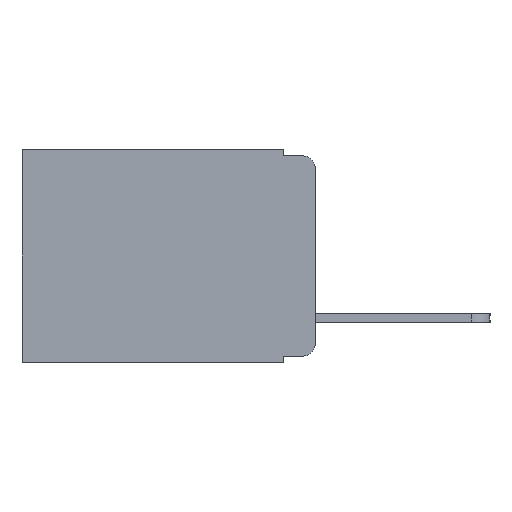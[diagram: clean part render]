
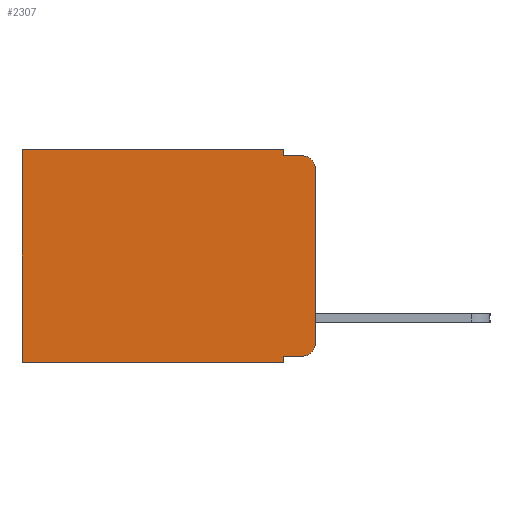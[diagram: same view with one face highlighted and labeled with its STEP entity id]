
A CAD part, left-side view. The second image highlights one B-rep face of the part: STEP entity #2307.
In plain terms, the highlighted planar face has unit normal (-1, 0, 0).
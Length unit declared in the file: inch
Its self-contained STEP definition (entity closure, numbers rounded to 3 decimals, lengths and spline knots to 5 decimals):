
#238 = CARTESIAN_POINT ( 'NONE',  ( 0.298, 0., 0. ) ) ;
#372 = VERTEX_POINT ( 'NONE', #7127 ) ;
#627 = DIRECTION ( 'NONE',  ( 0., 0., -1. ) ) ;
#700 = CARTESIAN_POINT ( 'NONE',  ( 0.298, 0.02, -0.03 ) ) ;
#803 = ORIENTED_EDGE ( 'NONE', *, *, #5936, .T. ) ;
#814 = EDGE_CURVE ( 'NONE', #4172, #1326, #2191, .T. ) ;
#929 = CARTESIAN_POINT ( 'NONE',  ( 0.298, 0.473, -0.343 ) ) ;
#932 = ORIENTED_EDGE ( 'NONE', *, *, #12882, .T. ) ;
#1138 = CARTESIAN_POINT ( 'NONE',  ( 0.298, 0.051, -0.333 ) ) ;
#1326 = VERTEX_POINT ( 'NONE', #11795 ) ;
#1337 = CIRCLE ( 'NONE', #1588, 0.02 ) ;
#1414 = VECTOR ( 'NONE', #9868, 39.37008 ) ;
#1460 = CARTESIAN_POINT ( 'NONE',  ( 0.298, 0.473, 0. ) ) ;
#1588 = AXIS2_PLACEMENT_3D ( 'NONE', #700, #6025, #6030 ) ;
#2191 = LINE ( 'NONE', #16276, #13257 ) ;
#2288 = EDGE_LOOP ( 'NONE', ( #4016, #4283, #4081, #4020, #5687, #7253, #7400, #7434, #803, #932 ) ) ;
#2307 = ADVANCED_FACE ( 'NONE', ( #2395 ), #15409, .F. ) ;
#2395 = FACE_OUTER_BOUND ( 'NONE', #2288, .T. ) ;
#2563 = VECTOR ( 'NONE', #11891, 39.37008 ) ;
#3158 = VECTOR ( 'NONE', #16912, 39.37008 ) ;
#3178 = VERTEX_POINT ( 'NONE', #10220 ) ;
#3566 = CARTESIAN_POINT ( 'NONE',  ( 0.298, 0.051, -0.01 ) ) ;
#3858 = VERTEX_POINT ( 'NONE', #9450 ) ;
#3864 = EDGE_CURVE ( 'NONE', #1326, #13881, #12593, .T. ) ;
#4016 = ORIENTED_EDGE ( 'NONE', *, *, #4179, .F. ) ;
#4020 = ORIENTED_EDGE ( 'NONE', *, *, #7780, .F. ) ;
#4081 = ORIENTED_EDGE ( 'NONE', *, *, #10175, .F. ) ;
#4172 = VERTEX_POINT ( 'NONE', #6106 ) ;
#4179 = EDGE_CURVE ( 'NONE', #15504, #3178, #4556, .T. ) ;
#4283 = ORIENTED_EDGE ( 'NONE', *, *, #5655, .T. ) ;
#4556 = LINE ( 'NONE', #9999, #7911 ) ;
#4930 = AXIS2_PLACEMENT_3D ( 'NONE', #238, #13393, #14440 ) ;
#5003 = DIRECTION ( 'NONE',  ( 0., 1., 0. ) ) ;
#5655 = EDGE_CURVE ( 'NONE', #15504, #3858, #1337, .T. ) ;
#5687 = ORIENTED_EDGE ( 'NONE', *, *, #814, .T. ) ;
#5936 = EDGE_CURVE ( 'NONE', #6296, #372, #6985, .T. ) ;
#6025 = DIRECTION ( 'NONE',  ( -1., 0., 0. ) ) ;
#6030 = DIRECTION ( 'NONE',  ( 0., 0., -1. ) ) ;
#6106 = CARTESIAN_POINT ( 'NONE',  ( 0.298, 0.051, 0. ) ) ;
#6243 = LINE ( 'NONE', #7939, #16553 ) ;
#6296 = VERTEX_POINT ( 'NONE', #1138 ) ;
#6985 = LINE ( 'NONE', #10076, #3158 ) ;
#7100 = EDGE_CURVE ( 'NONE', #6296, #12480, #15959, .T. ) ;
#7127 = CARTESIAN_POINT ( 'NONE',  ( 0.298, 0.02, -0.333 ) ) ;
#7253 = ORIENTED_EDGE ( 'NONE', *, *, #3864, .T. ) ;
#7400 = ORIENTED_EDGE ( 'NONE', *, *, #15795, .F. ) ;
#7434 = ORIENTED_EDGE ( 'NONE', *, *, #7100, .F. ) ;
#7780 = EDGE_CURVE ( 'NONE', #4172, #11171, #6243, .T. ) ;
#7826 = DIRECTION ( 'NONE',  ( 0., 1., 0. ) ) ;
#7899 = CARTESIAN_POINT ( 'NONE',  ( 0.298, 0.051, 0. ) ) ;
#7911 = VECTOR ( 'NONE', #9103, 39.37008 ) ;
#7939 = CARTESIAN_POINT ( 'NONE',  ( 0.298, 0.051, 0. ) ) ;
#8819 = VECTOR ( 'NONE', #14677, 39.37008 ) ;
#9103 = DIRECTION ( 'NONE',  ( 0., 0., -1. ) ) ;
#9143 = DIRECTION ( 'NONE',  ( -1., 0., 0. ) ) ;
#9268 = DIRECTION ( 'NONE',  ( 0., 0., -1. ) ) ;
#9450 = CARTESIAN_POINT ( 'NONE',  ( 0.298, 0.02, -0.01 ) ) ;
#9868 = DIRECTION ( 'NONE',  ( 0., 0., -1. ) ) ;
#9999 = CARTESIAN_POINT ( 'NONE',  ( 0.298, 0., 0. ) ) ;
#10076 = CARTESIAN_POINT ( 'NONE',  ( 0.298, 0.051, -0.333 ) ) ;
#10124 = CIRCLE ( 'NONE', #17299, 0.02 ) ;
#10175 = EDGE_CURVE ( 'NONE', #11171, #3858, #13995, .T. ) ;
#10220 = CARTESIAN_POINT ( 'NONE',  ( 0.298, 0., -0.313 ) ) ;
#11171 = VERTEX_POINT ( 'NONE', #11377 ) ;
#11377 = CARTESIAN_POINT ( 'NONE',  ( 0.298, 0.051, -0.01 ) ) ;
#11795 = CARTESIAN_POINT ( 'NONE',  ( 0.298, 0.473, 0. ) ) ;
#11891 = DIRECTION ( 'NONE',  ( 0., -1., 0. ) ) ;
#11909 = CARTESIAN_POINT ( 'NONE',  ( 0.298, 0., -0.343 ) ) ;
#12448 = CARTESIAN_POINT ( 'NONE',  ( 0.298, 0.051, -0.343 ) ) ;
#12480 = VERTEX_POINT ( 'NONE', #12448 ) ;
#12593 = LINE ( 'NONE', #1460, #1414 ) ;
#12729 = VECTOR ( 'NONE', #5003, 39.37008 ) ;
#12882 = EDGE_CURVE ( 'NONE', #372, #3178, #10124, .T. ) ;
#13140 = LINE ( 'NONE', #11909, #12729 ) ;
#13257 = VECTOR ( 'NONE', #7826, 39.37008 ) ;
#13393 = DIRECTION ( 'NONE',  ( 1., 0., 0. ) ) ;
#13881 = VERTEX_POINT ( 'NONE', #929 ) ;
#13995 = LINE ( 'NONE', #3566, #2563 ) ;
#14440 = DIRECTION ( 'NONE',  ( 0., 0., -1. ) ) ;
#14677 = DIRECTION ( 'NONE',  ( 0., 0., -1. ) ) ;
#15393 = CARTESIAN_POINT ( 'NONE',  ( 0.298, 0., -0.03 ) ) ;
#15409 = PLANE ( 'NONE',  #4930 ) ;
#15504 = VERTEX_POINT ( 'NONE', #15393 ) ;
#15795 = EDGE_CURVE ( 'NONE', #12480, #13881, #13140, .T. ) ;
#15959 = LINE ( 'NONE', #7899, #8819 ) ;
#16276 = CARTESIAN_POINT ( 'NONE',  ( 0.298, 0., 0. ) ) ;
#16553 = VECTOR ( 'NONE', #9268, 39.37008 ) ;
#16912 = DIRECTION ( 'NONE',  ( 0., -1., 0. ) ) ;
#17145 = CARTESIAN_POINT ( 'NONE',  ( 0.298, 0.02, -0.313 ) ) ;
#17299 = AXIS2_PLACEMENT_3D ( 'NONE', #17145, #9143, #627 ) ;
